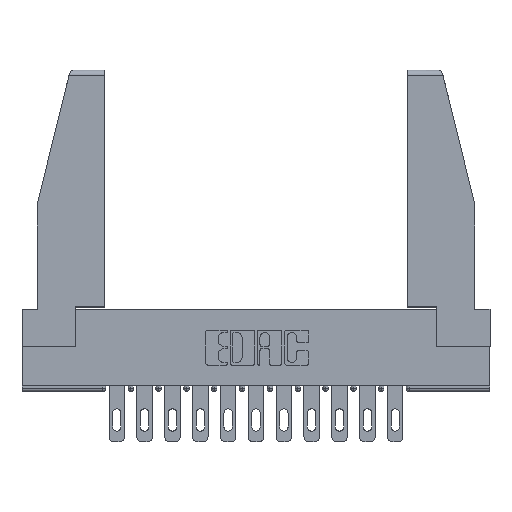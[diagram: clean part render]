
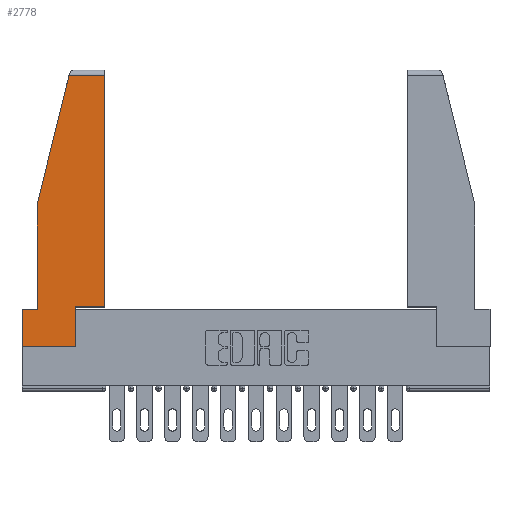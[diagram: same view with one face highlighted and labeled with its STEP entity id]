
A CAD part, top view. The second image highlights one B-rep face of the part: STEP entity #2778.
In plain terms, the highlighted planar face has unit normal (0, 0, 1).
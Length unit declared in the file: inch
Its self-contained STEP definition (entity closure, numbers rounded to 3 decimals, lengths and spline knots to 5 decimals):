
#64 = VERTEX_POINT ( 'NONE', #2224 ) ;
#199 = CARTESIAN_POINT ( 'NONE',  ( 0.461, 0.223, 0. ) ) ;
#539 = VECTOR ( 'NONE', #3507, 39.37008 ) ;
#809 = VERTEX_POINT ( 'NONE', #5042 ) ;
#1512 = LINE ( 'NONE', #8006, #8443 ) ;
#1553 = VERTEX_POINT ( 'NONE', #12316 ) ;
#1750 = CARTESIAN_POINT ( 'NONE',  ( 0.086, 0.21, 0. ) ) ;
#1848 = DIRECTION ( 'NONE',  ( -1., 0., 0. ) ) ;
#2224 = CARTESIAN_POINT ( 'NONE',  ( 0.086, 0.8, 0. ) ) ;
#2267 = LINE ( 'NONE', #7629, #15913 ) ;
#2401 = LINE ( 'NONE', #10009, #539 ) ;
#2621 = CARTESIAN_POINT ( 'NONE',  ( 0.086, 0.8, 0. ) ) ;
#2655 = VECTOR ( 'NONE', #1848, 39.37008 ) ;
#2778 = ADVANCED_FACE ( 'NONE', ( #16106 ), #12661, .T. ) ;
#2893 = AXIS2_PLACEMENT_3D ( 'NONE', #4464, #14924, #15331 ) ;
#2923 = VERTEX_POINT ( 'NONE', #3666 ) ;
#3125 = LINE ( 'NONE', #8338, #2655 ) ;
#3192 = CARTESIAN_POINT ( 'NONE',  ( 0.461, 0.223, 0. ) ) ;
#3466 = EDGE_CURVE ( 'NONE', #809, #11916, #1512, .T. ) ;
#3507 = DIRECTION ( 'NONE',  ( 1., 0., 0. ) ) ;
#3641 = ORIENTED_EDGE ( 'NONE', *, *, #14314, .T. ) ;
#3666 = CARTESIAN_POINT ( 'NONE',  ( 0.461, 1.52, 0. ) ) ;
#3935 = ORIENTED_EDGE ( 'NONE', *, *, #11957, .T. ) ;
#4246 = ORIENTED_EDGE ( 'NONE', *, *, #6744, .T. ) ;
#4464 = CARTESIAN_POINT ( 'NONE',  ( 0., 0., 0. ) ) ;
#5042 = CARTESIAN_POINT ( 'NONE',  ( 0.297, 0.223, 0. ) ) ;
#5157 = EDGE_CURVE ( 'NONE', #6858, #64, #8065, .T. ) ;
#5243 = DIRECTION ( 'NONE',  ( 1., 0., 0. ) ) ;
#5692 = CARTESIAN_POINT ( 'NONE',  ( 0., 0.21, 0. ) ) ;
#6744 = EDGE_CURVE ( 'NONE', #2923, #6858, #3125, .T. ) ;
#6751 = ORIENTED_EDGE ( 'NONE', *, *, #3466, .T. ) ;
#6858 = VERTEX_POINT ( 'NONE', #11260 ) ;
#7112 = VERTEX_POINT ( 'NONE', #1750 ) ;
#7390 = EDGE_LOOP ( 'NONE', ( #10070, #4246, #9612, #11668, #7458, #3935, #3641, #13086, #6751 ) ) ;
#7458 = ORIENTED_EDGE ( 'NONE', *, *, #11268, .T. ) ;
#7588 = VECTOR ( 'NONE', #9355, 39.37008 ) ;
#7629 = CARTESIAN_POINT ( 'NONE',  ( 0., 0.21, 0. ) ) ;
#7860 = CARTESIAN_POINT ( 'NONE',  ( 0.297, 0., 0. ) ) ;
#8006 = CARTESIAN_POINT ( 'NONE',  ( 0.297, 0.223, 0. ) ) ;
#8065 = LINE ( 'NONE', #10625, #7588 ) ;
#8338 = CARTESIAN_POINT ( 'NONE',  ( 0., 1.52, 0. ) ) ;
#8375 = EDGE_CURVE ( 'NONE', #11916, #2923, #9613, .T. ) ;
#8443 = VECTOR ( 'NONE', #5243, 39.37008 ) ;
#8446 = VECTOR ( 'NONE', #15272, 39.37008 ) ;
#8947 = VERTEX_POINT ( 'NONE', #14221 ) ;
#9325 = DIRECTION ( 'NONE',  ( 0., 1., 0. ) ) ;
#9355 = DIRECTION ( 'NONE',  ( -0.239, -0.971, 0. ) ) ;
#9612 = ORIENTED_EDGE ( 'NONE', *, *, #5157, .T. ) ;
#9613 = LINE ( 'NONE', #3192, #8446 ) ;
#9824 = DIRECTION ( 'NONE',  ( 0., -1., 0. ) ) ;
#10009 = CARTESIAN_POINT ( 'NONE',  ( 0., 0., 0. ) ) ;
#10070 = ORIENTED_EDGE ( 'NONE', *, *, #8375, .T. ) ;
#10625 = CARTESIAN_POINT ( 'NONE',  ( 0.271, 1.55, 0. ) ) ;
#10736 = VECTOR ( 'NONE', #15558, 39.37008 ) ;
#11015 = VECTOR ( 'NONE', #9824, 39.37008 ) ;
#11260 = CARTESIAN_POINT ( 'NONE',  ( 0.2636, 1.52, 0. ) ) ;
#11268 = EDGE_CURVE ( 'NONE', #7112, #11389, #2267, .T. ) ;
#11389 = VERTEX_POINT ( 'NONE', #12782 ) ;
#11535 = LINE ( 'NONE', #2621, #10736 ) ;
#11668 = ORIENTED_EDGE ( 'NONE', *, *, #12112, .T. ) ;
#11916 = VERTEX_POINT ( 'NONE', #199 ) ;
#11939 = EDGE_CURVE ( 'NONE', #8947, #809, #13096, .T. ) ;
#11957 = EDGE_CURVE ( 'NONE', #11389, #1553, #15405, .T. ) ;
#12112 = EDGE_CURVE ( 'NONE', #64, #7112, #11535, .T. ) ;
#12316 = CARTESIAN_POINT ( 'NONE',  ( 0., 0., 0. ) ) ;
#12661 = PLANE ( 'NONE',  #2893 ) ;
#12782 = CARTESIAN_POINT ( 'NONE',  ( 0., 0.21, 0. ) ) ;
#13086 = ORIENTED_EDGE ( 'NONE', *, *, #11939, .T. ) ;
#13096 = LINE ( 'NONE', #7860, #13753 ) ;
#13753 = VECTOR ( 'NONE', #9325, 39.37008 ) ;
#13998 = DIRECTION ( 'NONE',  ( -1., 0., 0. ) ) ;
#14221 = CARTESIAN_POINT ( 'NONE',  ( 0.297, 0., 0. ) ) ;
#14314 = EDGE_CURVE ( 'NONE', #1553, #8947, #2401, .T. ) ;
#14924 = DIRECTION ( 'NONE',  ( 0., 0., 1. ) ) ;
#15272 = DIRECTION ( 'NONE',  ( 0., 1., 0. ) ) ;
#15331 = DIRECTION ( 'NONE',  ( 1., 0., 0. ) ) ;
#15405 = LINE ( 'NONE', #5692, #11015 ) ;
#15558 = DIRECTION ( 'NONE',  ( 0., -1., 0. ) ) ;
#15913 = VECTOR ( 'NONE', #13998, 39.37008 ) ;
#16106 = FACE_OUTER_BOUND ( 'NONE', #7390, .T. ) ;
